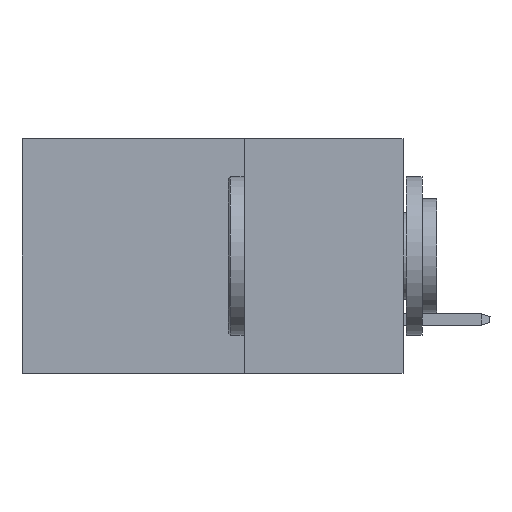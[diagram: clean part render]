
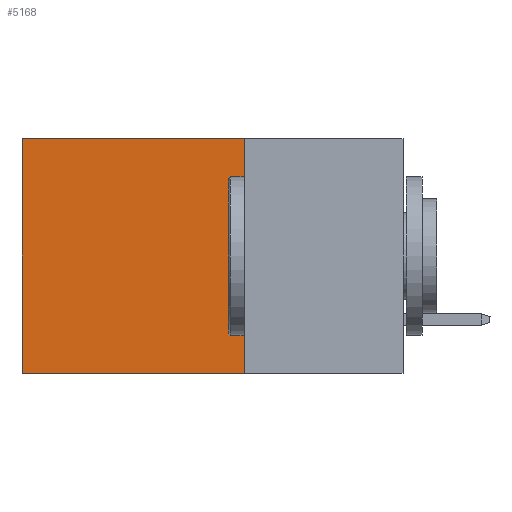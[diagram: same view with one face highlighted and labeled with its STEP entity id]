
A CAD part, left-side view. The second image highlights one B-rep face of the part: STEP entity #5168.
In plain terms, the highlighted planar face has unit normal (-1, 0, 0).
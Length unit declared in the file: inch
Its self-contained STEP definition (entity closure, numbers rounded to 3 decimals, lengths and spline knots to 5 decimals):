
#10 = CARTESIAN_POINT ( 'NONE',  ( 0.2875, 0.25, 0. ) ) ;
#3401 = ORIENTED_EDGE ( 'NONE', *, *, #22676, .T. ) ;
#3550 = AXIS2_PLACEMENT_3D ( 'NONE', #10, #6126, #17718 ) ;
#4282 = CARTESIAN_POINT ( 'NONE',  ( 0.2875, 0.6, -0.37 ) ) ;
#5088 = EDGE_CURVE ( 'NONE', #5499, #6055, #10791, .T. ) ;
#5168 = ADVANCED_FACE ( 'NONE', ( #15101 ), #13231, .F. ) ;
#5499 = VERTEX_POINT ( 'NONE', #6641 ) ;
#5815 = CARTESIAN_POINT ( 'NONE',  ( 0.2875, 0.6, 0. ) ) ;
#5950 = ORIENTED_EDGE ( 'NONE', *, *, #26900, .F. ) ;
#6055 = VERTEX_POINT ( 'NONE', #4282 ) ;
#6126 = DIRECTION ( 'NONE',  ( 1., 0., 0. ) ) ;
#6641 = CARTESIAN_POINT ( 'NONE',  ( 0.2875, 0.25, -0.37 ) ) ;
#6940 = LINE ( 'NONE', #19827, #27551 ) ;
#8990 = DIRECTION ( 'NONE',  ( 0., 0., -1. ) ) ;
#9398 = EDGE_LOOP ( 'NONE', ( #3401, #18643, #5950, #24507 ) ) ;
#10775 = CARTESIAN_POINT ( 'NONE',  ( 0.2875, 0.6, 0. ) ) ;
#10791 = LINE ( 'NONE', #12955, #24330 ) ;
#12150 = VERTEX_POINT ( 'NONE', #5815 ) ;
#12258 = CARTESIAN_POINT ( 'NONE',  ( 0.2875, 0.25, 0. ) ) ;
#12542 = DIRECTION ( 'NONE',  ( 0., 1., 0. ) ) ;
#12955 = CARTESIAN_POINT ( 'NONE',  ( 0.2875, 0.25, -0.37 ) ) ;
#13231 = PLANE ( 'NONE',  #3550 ) ;
#15086 = LINE ( 'NONE', #10775, #18623 ) ;
#15101 = FACE_OUTER_BOUND ( 'NONE', #9398, .T. ) ;
#16850 = DIRECTION ( 'NONE',  ( 0., 0., -1. ) ) ;
#17136 = CARTESIAN_POINT ( 'NONE',  ( 0.2875, 0.25, 0. ) ) ;
#17563 = EDGE_CURVE ( 'NONE', #19268, #12150, #25677, .T. ) ;
#17718 = DIRECTION ( 'NONE',  ( 0., 0., -1. ) ) ;
#18623 = VECTOR ( 'NONE', #16850, 39.37008 ) ;
#18643 = ORIENTED_EDGE ( 'NONE', *, *, #5088, .F. ) ;
#19268 = VERTEX_POINT ( 'NONE', #17136 ) ;
#19827 = CARTESIAN_POINT ( 'NONE',  ( 0.2875, 0.25, 0. ) ) ;
#22676 = EDGE_CURVE ( 'NONE', #12150, #6055, #15086, .T. ) ;
#24330 = VECTOR ( 'NONE', #26226, 39.37008 ) ;
#24507 = ORIENTED_EDGE ( 'NONE', *, *, #17563, .T. ) ;
#25677 = LINE ( 'NONE', #12258, #27725 ) ;
#26226 = DIRECTION ( 'NONE',  ( 0., 1., 0. ) ) ;
#26900 = EDGE_CURVE ( 'NONE', #19268, #5499, #6940, .T. ) ;
#27551 = VECTOR ( 'NONE', #8990, 39.37008 ) ;
#27725 = VECTOR ( 'NONE', #12542, 39.37008 ) ;
